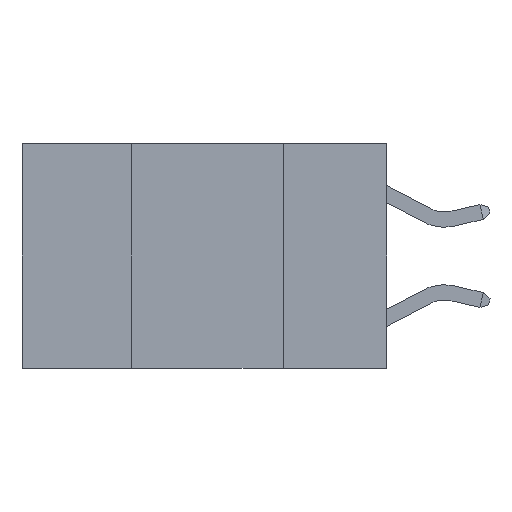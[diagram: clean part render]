
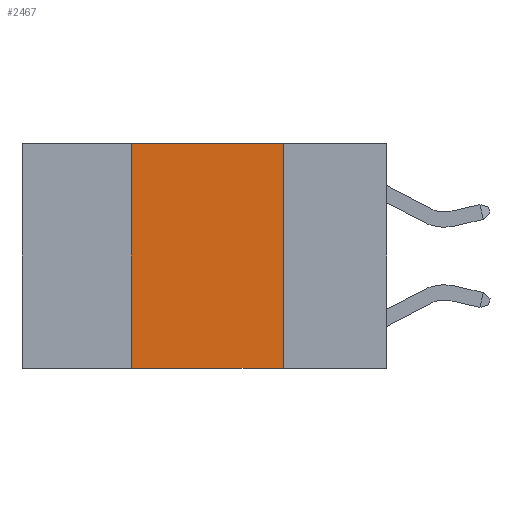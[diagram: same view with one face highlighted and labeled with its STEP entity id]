
A CAD part, left-side view. The second image highlights one B-rep face of the part: STEP entity #2467.
In plain terms, the highlighted planar face has unit normal (-1, 0, 0).
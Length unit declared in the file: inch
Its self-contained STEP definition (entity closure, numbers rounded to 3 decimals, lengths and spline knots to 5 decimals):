
#720 = ORIENTED_EDGE ( 'NONE', *, *, #10004, .F. ) ;
#1124 = DIRECTION ( 'NONE',  ( 0., 0., -1. ) ) ;
#1157 = LINE ( 'NONE', #6574, #10125 ) ;
#1361 = DIRECTION ( 'NONE',  ( 0., -1., 0. ) ) ;
#2467 = ADVANCED_FACE ( 'NONE', ( #2792 ), #11103, .F. ) ;
#2484 = ORIENTED_EDGE ( 'NONE', *, *, #10712, .F. ) ;
#2715 = VECTOR ( 'NONE', #10810, 39.37008 ) ;
#2792 = FACE_OUTER_BOUND ( 'NONE', #10197, .T. ) ;
#3041 = ORIENTED_EDGE ( 'NONE', *, *, #5964, .F. ) ;
#3195 = CARTESIAN_POINT ( 'NONE',  ( 0., 0.42, 0. ) ) ;
#4207 = VECTOR ( 'NONE', #1124, 39.37008 ) ;
#4447 = VERTEX_POINT ( 'NONE', #11038 ) ;
#4593 = CARTESIAN_POINT ( 'NONE',  ( 0., 0.6, 0. ) ) ;
#4644 = CARTESIAN_POINT ( 'NONE',  ( 0., 0.6, 0. ) ) ;
#4735 = LINE ( 'NONE', #4936, #2715 ) ;
#4936 = CARTESIAN_POINT ( 'NONE',  ( 0., 0.42, 0. ) ) ;
#5053 = VECTOR ( 'NONE', #7991, 39.37008 ) ;
#5480 = DIRECTION ( 'NONE',  ( 1., 0., 0. ) ) ;
#5964 = EDGE_CURVE ( 'NONE', #11440, #4447, #9289, .T. ) ;
#6574 = CARTESIAN_POINT ( 'NONE',  ( 0., 0.6, -0.37 ) ) ;
#7014 = VERTEX_POINT ( 'NONE', #9141 ) ;
#7142 = AXIS2_PLACEMENT_3D ( 'NONE', #4644, #5480, #11380 ) ;
#7991 = DIRECTION ( 'NONE',  ( 0., -1., 0. ) ) ;
#8197 = CARTESIAN_POINT ( 'NONE',  ( 0., 0.17, 0. ) ) ;
#9141 = CARTESIAN_POINT ( 'NONE',  ( 0., 0.42, -0.37 ) ) ;
#9289 = LINE ( 'NONE', #4593, #5053 ) ;
#9798 = ORIENTED_EDGE ( 'NONE', *, *, #11427, .T. ) ;
#10002 = CARTESIAN_POINT ( 'NONE',  ( 0., 0.17, -0.37 ) ) ;
#10004 = EDGE_CURVE ( 'NONE', #7014, #11440, #4735, .T. ) ;
#10014 = VERTEX_POINT ( 'NONE', #10002 ) ;
#10125 = VECTOR ( 'NONE', #1361, 39.37008 ) ;
#10197 = EDGE_LOOP ( 'NONE', ( #2484, #3041, #720, #9798 ) ) ;
#10712 = EDGE_CURVE ( 'NONE', #4447, #10014, #11154, .T. ) ;
#10810 = DIRECTION ( 'NONE',  ( 0., 0., 1. ) ) ;
#11038 = CARTESIAN_POINT ( 'NONE',  ( 0., 0.17, 0. ) ) ;
#11103 = PLANE ( 'NONE',  #7142 ) ;
#11154 = LINE ( 'NONE', #8197, #4207 ) ;
#11380 = DIRECTION ( 'NONE',  ( 0., 0., -1. ) ) ;
#11427 = EDGE_CURVE ( 'NONE', #7014, #10014, #1157, .T. ) ;
#11440 = VERTEX_POINT ( 'NONE', #3195 ) ;
